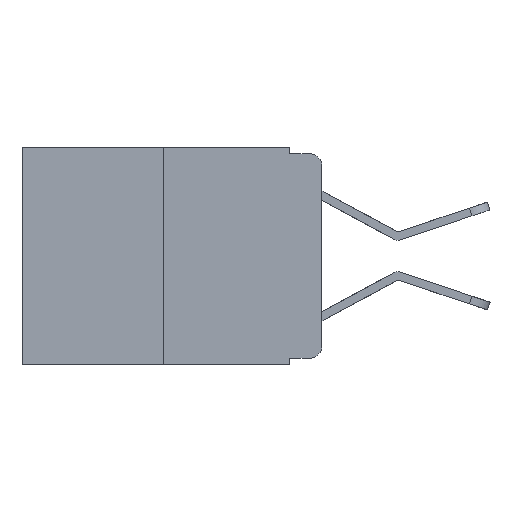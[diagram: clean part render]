
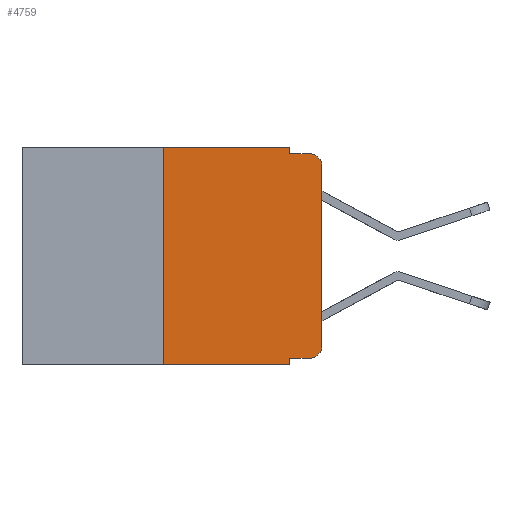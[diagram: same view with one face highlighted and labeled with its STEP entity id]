
A CAD part, left-side view. The second image highlights one B-rep face of the part: STEP entity #4759.
In plain terms, the highlighted planar face has unit normal (-1, 0, 0).
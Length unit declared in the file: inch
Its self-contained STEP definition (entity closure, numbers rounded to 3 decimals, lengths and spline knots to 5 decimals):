
#331 = VERTEX_POINT ( 'NONE', #20386 ) ;
#604 = AXIS2_PLACEMENT_3D ( 'NONE', #10645, #15101, #17129 ) ;
#650 = CIRCLE ( 'NONE', #17017, 0.02 ) ;
#771 = VERTEX_POINT ( 'NONE', #17191 ) ;
#797 = LINE ( 'NONE', #12237, #8340 ) ;
#879 = EDGE_CURVE ( 'NONE', #2544, #6404, #6505, .T. ) ;
#1180 = CARTESIAN_POINT ( 'NONE',  ( 0., 0., -0.03 ) ) ;
#1263 = CIRCLE ( 'NONE', #604, 0.02 ) ;
#1508 = EDGE_CURVE ( 'NONE', #2873, #771, #650, .T. ) ;
#1532 = VECTOR ( 'NONE', #20967, 39.37008 ) ;
#1932 = VECTOR ( 'NONE', #18641, 39.37008 ) ;
#2544 = VERTEX_POINT ( 'NONE', #13864 ) ;
#2873 = VERTEX_POINT ( 'NONE', #3396 ) ;
#3065 = VECTOR ( 'NONE', #9509, 39.37008 ) ;
#3119 = CARTESIAN_POINT ( 'NONE',  ( 0., 0.051, 0. ) ) ;
#3245 = CARTESIAN_POINT ( 'NONE',  ( 0., 0.02, -0.01 ) ) ;
#3396 = CARTESIAN_POINT ( 'NONE',  ( 0., 0.02, -0.333 ) ) ;
#3698 = LINE ( 'NONE', #17584, #3065 ) ;
#3723 = VERTEX_POINT ( 'NONE', #1180 ) ;
#4759 = ADVANCED_FACE ( 'NONE', ( #19263 ), #10996, .F. ) ;
#5391 = DIRECTION ( 'NONE',  ( -1., 0., 0. ) ) ;
#5645 = LINE ( 'NONE', #17167, #1932 ) ;
#6187 = ORIENTED_EDGE ( 'NONE', *, *, #17015, .F. ) ;
#6404 = VERTEX_POINT ( 'NONE', #18185 ) ;
#6505 = LINE ( 'NONE', #14615, #1532 ) ;
#6524 = VERTEX_POINT ( 'NONE', #8189 ) ;
#6527 = LINE ( 'NONE', #12926, #12634 ) ;
#6954 = ORIENTED_EDGE ( 'NONE', *, *, #879, .F. ) ;
#7148 = VECTOR ( 'NONE', #11758, 39.37008 ) ;
#8189 = CARTESIAN_POINT ( 'NONE',  ( 0., 0.051, 0. ) ) ;
#8340 = VECTOR ( 'NONE', #15202, 39.37008 ) ;
#8947 = VERTEX_POINT ( 'NONE', #17383 ) ;
#9200 = EDGE_CURVE ( 'NONE', #15335, #6404, #14298, .T. ) ;
#9343 = EDGE_CURVE ( 'NONE', #3723, #11952, #1263, .T. ) ;
#9509 = DIRECTION ( 'NONE',  ( 0., 0., 1. ) ) ;
#9625 = DIRECTION ( 'NONE',  ( 0., 0., -1. ) ) ;
#9654 = EDGE_LOOP ( 'NONE', ( #19791, #17207, #6187, #13527, #10985, #14279, #9806, #6954, #12754, #20289 ) ) ;
#9688 = DIRECTION ( 'NONE',  ( 0., 0., -1. ) ) ;
#9806 = ORIENTED_EDGE ( 'NONE', *, *, #9200, .T. ) ;
#9971 = EDGE_CURVE ( 'NONE', #6524, #8947, #17604, .T. ) ;
#10645 = CARTESIAN_POINT ( 'NONE',  ( 0., 0.02, -0.03 ) ) ;
#10985 = ORIENTED_EDGE ( 'NONE', *, *, #13694, .F. ) ;
#10996 = PLANE ( 'NONE',  #17922 ) ;
#11101 = CARTESIAN_POINT ( 'NONE',  ( 0., 0.473, -0.343 ) ) ;
#11485 = EDGE_CURVE ( 'NONE', #15335, #331, #3698, .T. ) ;
#11597 = DIRECTION ( 'NONE',  ( 0., -1., 0. ) ) ;
#11758 = DIRECTION ( 'NONE',  ( 0., -1., 0. ) ) ;
#11952 = VERTEX_POINT ( 'NONE', #3245 ) ;
#12237 = CARTESIAN_POINT ( 'NONE',  ( 0., 0.051, -0.01 ) ) ;
#12548 = EDGE_CURVE ( 'NONE', #2544, #2873, #15473, .T. ) ;
#12550 = VECTOR ( 'NONE', #9625, 39.37008 ) ;
#12634 = VECTOR ( 'NONE', #16553, 39.37008 ) ;
#12754 = ORIENTED_EDGE ( 'NONE', *, *, #12548, .T. ) ;
#12926 = CARTESIAN_POINT ( 'NONE',  ( 0., 0.473, 0. ) ) ;
#13527 = ORIENTED_EDGE ( 'NONE', *, *, #9971, .F. ) ;
#13571 = CARTESIAN_POINT ( 'NONE',  ( 0., 0.051, -0.333 ) ) ;
#13601 = DIRECTION ( 'NONE',  ( 0., 0., -1. ) ) ;
#13694 = EDGE_CURVE ( 'NONE', #331, #6524, #6527, .T. ) ;
#13864 = CARTESIAN_POINT ( 'NONE',  ( 0., 0.051, -0.333 ) ) ;
#14279 = ORIENTED_EDGE ( 'NONE', *, *, #11485, .F. ) ;
#14298 = LINE ( 'NONE', #11101, #18970 ) ;
#14615 = CARTESIAN_POINT ( 'NONE',  ( 0., 0.051, 0. ) ) ;
#15101 = DIRECTION ( 'NONE',  ( -1., 0., 0. ) ) ;
#15202 = DIRECTION ( 'NONE',  ( 0., -1., 0. ) ) ;
#15335 = VERTEX_POINT ( 'NONE', #18315 ) ;
#15473 = LINE ( 'NONE', #13571, #7148 ) ;
#15972 = DIRECTION ( 'NONE',  ( 1., 0., 0. ) ) ;
#16553 = DIRECTION ( 'NONE',  ( 0., -1., 0. ) ) ;
#16698 = CARTESIAN_POINT ( 'NONE',  ( 0., 0.02, -0.313 ) ) ;
#17015 = EDGE_CURVE ( 'NONE', #8947, #11952, #797, .T. ) ;
#17017 = AXIS2_PLACEMENT_3D ( 'NONE', #16698, #5391, #13601 ) ;
#17129 = DIRECTION ( 'NONE',  ( 0., 0., -1. ) ) ;
#17167 = CARTESIAN_POINT ( 'NONE',  ( 0., 0., 0. ) ) ;
#17191 = CARTESIAN_POINT ( 'NONE',  ( 0., 0., -0.313 ) ) ;
#17207 = ORIENTED_EDGE ( 'NONE', *, *, #9343, .T. ) ;
#17383 = CARTESIAN_POINT ( 'NONE',  ( 0., 0.051, -0.01 ) ) ;
#17584 = CARTESIAN_POINT ( 'NONE',  ( 0., 0.25, 0. ) ) ;
#17604 = LINE ( 'NONE', #3119, #12550 ) ;
#17922 = AXIS2_PLACEMENT_3D ( 'NONE', #19471, #15972, #9688 ) ;
#18185 = CARTESIAN_POINT ( 'NONE',  ( 0., 0.051, -0.343 ) ) ;
#18315 = CARTESIAN_POINT ( 'NONE',  ( 0., 0.25, -0.343 ) ) ;
#18641 = DIRECTION ( 'NONE',  ( 0., 0., 1. ) ) ;
#18970 = VECTOR ( 'NONE', #11597, 39.37008 ) ;
#19263 = FACE_OUTER_BOUND ( 'NONE', #9654, .T. ) ;
#19471 = CARTESIAN_POINT ( 'NONE',  ( 0., 0.473, 0. ) ) ;
#19577 = EDGE_CURVE ( 'NONE', #771, #3723, #5645, .T. ) ;
#19791 = ORIENTED_EDGE ( 'NONE', *, *, #19577, .T. ) ;
#20289 = ORIENTED_EDGE ( 'NONE', *, *, #1508, .T. ) ;
#20386 = CARTESIAN_POINT ( 'NONE',  ( 0., 0.25, 0. ) ) ;
#20967 = DIRECTION ( 'NONE',  ( 0., 0., -1. ) ) ;
